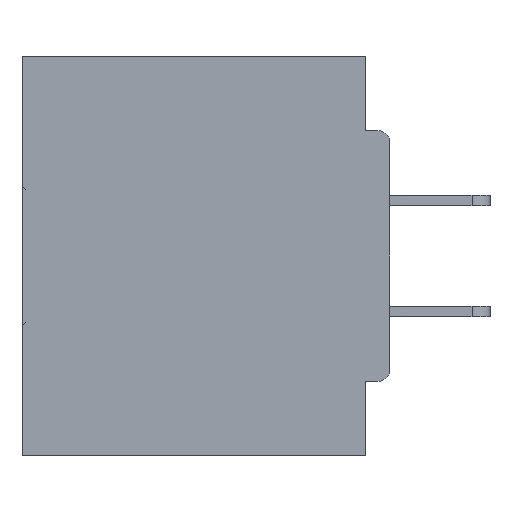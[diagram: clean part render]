
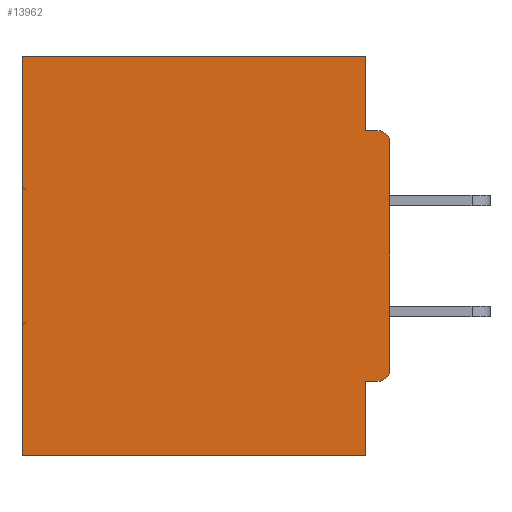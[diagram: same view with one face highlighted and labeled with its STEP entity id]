
A CAD part, left-side view. The second image highlights one B-rep face of the part: STEP entity #13962.
In plain terms, the highlighted planar face has unit normal (-1, 0, 0).
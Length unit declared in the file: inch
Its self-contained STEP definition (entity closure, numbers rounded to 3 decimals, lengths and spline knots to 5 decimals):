
#1102 = VECTOR ( 'NONE', #38322, 39.37008 ) ;
#1389 = AXIS2_PLACEMENT_3D ( 'NONE', #26399, #36669, #18762 ) ;
#2020 = DIRECTION ( 'NONE',  ( 0., -1., 0. ) ) ;
#2108 = CARTESIAN_POINT ( 'NONE',  ( 0.298, 0.031, -0.4065 ) ) ;
#2353 = VERTEX_POINT ( 'NONE', #6076 ) ;
#3872 = ORIENTED_EDGE ( 'NONE', *, *, #28711, .F. ) ;
#5060 = CARTESIAN_POINT ( 'NONE',  ( 0.298, 0., -0.0935 ) ) ;
#5065 = ORIENTED_EDGE ( 'NONE', *, *, #38695, .F. ) ;
#5104 = VECTOR ( 'NONE', #2020, 39.37008 ) ;
#5847 = CARTESIAN_POINT ( 'NONE',  ( 0.298, 0., 0. ) ) ;
#6076 = CARTESIAN_POINT ( 'NONE',  ( 0.298, 0., -0.3915 ) ) ;
#6328 = EDGE_CURVE ( 'NONE', #26656, #11768, #41417, .T. ) ;
#7011 = VERTEX_POINT ( 'NONE', #42596 ) ;
#7124 = CARTESIAN_POINT ( 'NONE',  ( 0.298, 0., -0.4065 ) ) ;
#7423 = EDGE_CURVE ( 'NONE', #14092, #2353, #27728, .T. ) ;
#9728 = CARTESIAN_POINT ( 'NONE',  ( 0.298, 0.031, -0.0935 ) ) ;
#10373 = VECTOR ( 'NONE', #36907, 39.37008 ) ;
#10744 = EDGE_LOOP ( 'NONE', ( #29636, #5065, #19413, #25870, #22718, #18891, #3872, #14013, #11507, #11925 ) ) ;
#10764 = VERTEX_POINT ( 'NONE', #33796 ) ;
#11439 = LINE ( 'NONE', #7124, #14175 ) ;
#11507 = ORIENTED_EDGE ( 'NONE', *, *, #7423, .T. ) ;
#11768 = VERTEX_POINT ( 'NONE', #36464 ) ;
#11925 = ORIENTED_EDGE ( 'NONE', *, *, #12991, .F. ) ;
#12886 = CARTESIAN_POINT ( 'NONE',  ( 0.298, 0.031, -0.5 ) ) ;
#12991 = EDGE_CURVE ( 'NONE', #7011, #2353, #27226, .T. ) ;
#13962 = ADVANCED_FACE ( 'NONE', ( #21632 ), #21268, .F. ) ;
#14013 = ORIENTED_EDGE ( 'NONE', *, *, #32813, .F. ) ;
#14092 = VERTEX_POINT ( 'NONE', #32272 ) ;
#14175 = VECTOR ( 'NONE', #35283, 39.37008 ) ;
#15277 = VECTOR ( 'NONE', #20030, 39.37008 ) ;
#17150 = DIRECTION ( 'NONE',  ( 1., 0., 0. ) ) ;
#17963 = LINE ( 'NONE', #34849, #34453 ) ;
#18762 = DIRECTION ( 'NONE',  ( 0., 0., -1. ) ) ;
#18891 = ORIENTED_EDGE ( 'NONE', *, *, #39846, .F. ) ;
#19045 = VERTEX_POINT ( 'NONE', #2108 ) ;
#19413 = ORIENTED_EDGE ( 'NONE', *, *, #32775, .F. ) ;
#19589 = CARTESIAN_POINT ( 'NONE',  ( 0.298, 0.031, 0. ) ) ;
#20030 = DIRECTION ( 'NONE',  ( 0., 0., -1. ) ) ;
#20978 = DIRECTION ( 'NONE',  ( 0., 0., -1. ) ) ;
#21051 = DIRECTION ( 'NONE',  ( 0., 1., 0. ) ) ;
#21268 = PLANE ( 'NONE',  #30489 ) ;
#21632 = FACE_OUTER_BOUND ( 'NONE', #10744, .T. ) ;
#21796 = LINE ( 'NONE', #35003, #39272 ) ;
#22718 = ORIENTED_EDGE ( 'NONE', *, *, #6328, .T. ) ;
#23257 = EDGE_CURVE ( 'NONE', #7011, #10764, #42019, .T. ) ;
#23638 = VERTEX_POINT ( 'NONE', #9728 ) ;
#24599 = EDGE_CURVE ( 'NONE', #28735, #26656, #25244, .T. ) ;
#24743 = CARTESIAN_POINT ( 'NONE',  ( 0.298, 0., 0. ) ) ;
#24842 = CARTESIAN_POINT ( 'NONE',  ( 0.298, 0.46, 0. ) ) ;
#25244 = LINE ( 'NONE', #42347, #33504 ) ;
#25870 = ORIENTED_EDGE ( 'NONE', *, *, #24599, .T. ) ;
#26399 = CARTESIAN_POINT ( 'NONE',  ( 0.298, 0.015, -0.3915 ) ) ;
#26656 = VERTEX_POINT ( 'NONE', #24842 ) ;
#27006 = DIRECTION ( 'NONE',  ( 0., 0., -1. ) ) ;
#27226 = LINE ( 'NONE', #5847, #10373 ) ;
#27728 = CIRCLE ( 'NONE', #1389, 0.015 ) ;
#27910 = DIRECTION ( 'NONE',  ( 0., 0., -1. ) ) ;
#28041 = CARTESIAN_POINT ( 'NONE',  ( 0.298, 0.015, -0.1085 ) ) ;
#28711 = EDGE_CURVE ( 'NONE', #19045, #42914, #41980, .T. ) ;
#28735 = VERTEX_POINT ( 'NONE', #19589 ) ;
#29489 = CARTESIAN_POINT ( 'NONE',  ( 0.298, 0.031, -0.5 ) ) ;
#29636 = ORIENTED_EDGE ( 'NONE', *, *, #23257, .T. ) ;
#30489 = AXIS2_PLACEMENT_3D ( 'NONE', #24743, #17150, #20978 ) ;
#31230 = LINE ( 'NONE', #5060, #5104 ) ;
#31451 = DIRECTION ( 'NONE',  ( -1., 0., 0. ) ) ;
#32272 = CARTESIAN_POINT ( 'NONE',  ( 0.298, 0.015, -0.4065 ) ) ;
#32775 = EDGE_CURVE ( 'NONE', #28735, #23638, #17963, .T. ) ;
#32813 = EDGE_CURVE ( 'NONE', #14092, #19045, #11439, .T. ) ;
#33504 = VECTOR ( 'NONE', #21051, 39.37008 ) ;
#33796 = CARTESIAN_POINT ( 'NONE',  ( 0.298, 0.015, -0.0935 ) ) ;
#34237 = AXIS2_PLACEMENT_3D ( 'NONE', #28041, #31451, #27006 ) ;
#34453 = VECTOR ( 'NONE', #27910, 39.37008 ) ;
#34849 = CARTESIAN_POINT ( 'NONE',  ( 0.298, 0.031, -0.5 ) ) ;
#35003 = CARTESIAN_POINT ( 'NONE',  ( 0.298, 0., -0.5 ) ) ;
#35283 = DIRECTION ( 'NONE',  ( 0., 1., 0. ) ) ;
#36464 = CARTESIAN_POINT ( 'NONE',  ( 0.298, 0.46, -0.5 ) ) ;
#36669 = DIRECTION ( 'NONE',  ( -1., 0., 0. ) ) ;
#36907 = DIRECTION ( 'NONE',  ( 0., 0., -1. ) ) ;
#38322 = DIRECTION ( 'NONE',  ( 0., 0., -1. ) ) ;
#38609 = DIRECTION ( 'NONE',  ( 0., 1., 0. ) ) ;
#38612 = CARTESIAN_POINT ( 'NONE',  ( 0.298, 0.46, 0. ) ) ;
#38695 = EDGE_CURVE ( 'NONE', #23638, #10764, #31230, .T. ) ;
#39272 = VECTOR ( 'NONE', #38609, 39.37008 ) ;
#39846 = EDGE_CURVE ( 'NONE', #42914, #11768, #21796, .T. ) ;
#41417 = LINE ( 'NONE', #38612, #1102 ) ;
#41980 = LINE ( 'NONE', #12886, #15277 ) ;
#42019 = CIRCLE ( 'NONE', #34237, 0.015 ) ;
#42347 = CARTESIAN_POINT ( 'NONE',  ( 0.298, 0., 0. ) ) ;
#42596 = CARTESIAN_POINT ( 'NONE',  ( 0.298, 0., -0.1085 ) ) ;
#42914 = VERTEX_POINT ( 'NONE', #29489 ) ;
